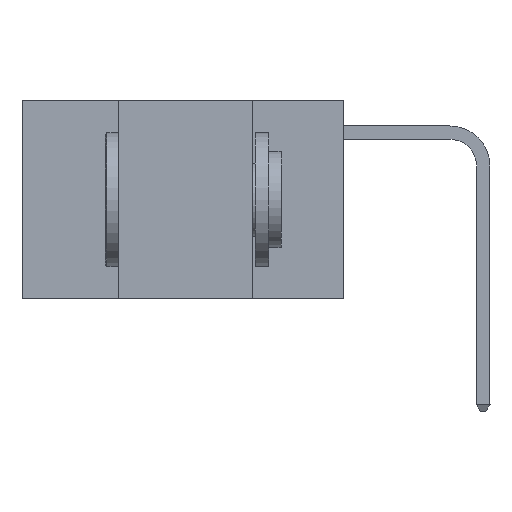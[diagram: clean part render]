
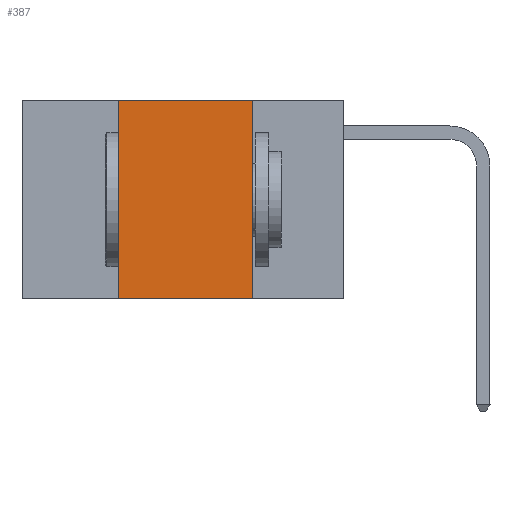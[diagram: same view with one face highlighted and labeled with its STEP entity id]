
A CAD part, left-side view. The second image highlights one B-rep face of the part: STEP entity #387.
In plain terms, the highlighted planar face has unit normal (-1, 0, 0).
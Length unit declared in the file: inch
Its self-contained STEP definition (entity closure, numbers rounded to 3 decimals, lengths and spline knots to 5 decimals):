
#106 = CARTESIAN_POINT ( 'NONE',  ( 0., 0.42, 0. ) ) ;
#387 = ADVANCED_FACE ( 'NONE', ( #13117 ), #16728, .F. ) ;
#1953 = CARTESIAN_POINT ( 'NONE',  ( 0., 0.17, 0. ) ) ;
#3826 = CARTESIAN_POINT ( 'NONE',  ( 0., 0.17, -0.37 ) ) ;
#3947 = VECTOR ( 'NONE', #16074, 39.37008 ) ;
#4049 = LINE ( 'NONE', #4574, #3947 ) ;
#4574 = CARTESIAN_POINT ( 'NONE',  ( 0., 0.17, 0. ) ) ;
#4590 = CARTESIAN_POINT ( 'NONE',  ( 0., 0.42, -0.37 ) ) ;
#4994 = DIRECTION ( 'NONE',  ( 0., -1., 0. ) ) ;
#5206 = EDGE_CURVE ( 'NONE', #15273, #10756, #4049, .T. ) ;
#6067 = EDGE_CURVE ( 'NONE', #11642, #15273, #14318, .T. ) ;
#6089 = DIRECTION ( 'NONE',  ( 0., 0., 1. ) ) ;
#6518 = VERTEX_POINT ( 'NONE', #4590 ) ;
#6908 = EDGE_LOOP ( 'NONE', ( #10420, #10444, #10526, #10614 ) ) ;
#8794 = LINE ( 'NONE', #14037, #11846 ) ;
#9753 = AXIS2_PLACEMENT_3D ( 'NONE', #15112, #14100, #10241 ) ;
#10183 = CARTESIAN_POINT ( 'NONE',  ( 0., 0.6, 0. ) ) ;
#10241 = DIRECTION ( 'NONE',  ( 0., 0., -1. ) ) ;
#10420 = ORIENTED_EDGE ( 'NONE', *, *, #5206, .F. ) ;
#10444 = ORIENTED_EDGE ( 'NONE', *, *, #6067, .F. ) ;
#10526 = ORIENTED_EDGE ( 'NONE', *, *, #14131, .F. ) ;
#10614 = ORIENTED_EDGE ( 'NONE', *, *, #13288, .T. ) ;
#10756 = VERTEX_POINT ( 'NONE', #3826 ) ;
#11363 = VECTOR ( 'NONE', #4994, 39.37008 ) ;
#11642 = VERTEX_POINT ( 'NONE', #106 ) ;
#11816 = LINE ( 'NONE', #13800, #12223 ) ;
#11846 = VECTOR ( 'NONE', #15313, 39.37008 ) ;
#12223 = VECTOR ( 'NONE', #6089, 39.37008 ) ;
#13117 = FACE_OUTER_BOUND ( 'NONE', #6908, .T. ) ;
#13288 = EDGE_CURVE ( 'NONE', #6518, #10756, #8794, .T. ) ;
#13800 = CARTESIAN_POINT ( 'NONE',  ( 0., 0.42, 0. ) ) ;
#14037 = CARTESIAN_POINT ( 'NONE',  ( 0., 0.6, -0.37 ) ) ;
#14100 = DIRECTION ( 'NONE',  ( 1., 0., 0. ) ) ;
#14131 = EDGE_CURVE ( 'NONE', #6518, #11642, #11816, .T. ) ;
#14318 = LINE ( 'NONE', #10183, #11363 ) ;
#15112 = CARTESIAN_POINT ( 'NONE',  ( 0., 0.6, 0. ) ) ;
#15273 = VERTEX_POINT ( 'NONE', #1953 ) ;
#15313 = DIRECTION ( 'NONE',  ( 0., -1., 0. ) ) ;
#16074 = DIRECTION ( 'NONE',  ( 0., 0., -1. ) ) ;
#16728 = PLANE ( 'NONE',  #9753 ) ;
